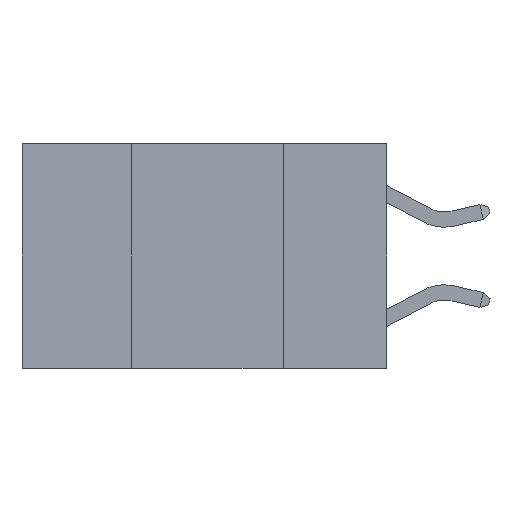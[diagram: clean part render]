
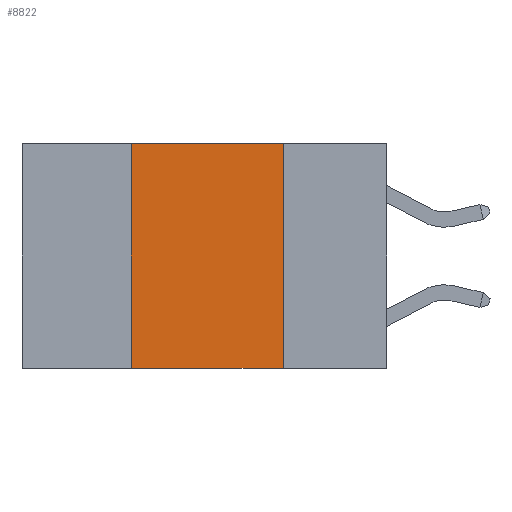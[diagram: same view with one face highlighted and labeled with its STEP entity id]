
A CAD part, left-side view. The second image highlights one B-rep face of the part: STEP entity #8822.
In plain terms, the highlighted planar face has unit normal (-1, 0, 0).
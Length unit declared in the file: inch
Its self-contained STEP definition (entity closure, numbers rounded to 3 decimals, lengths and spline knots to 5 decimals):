
#133 = DIRECTION ( 'NONE',  ( 0., 0., -1. ) ) ;
#435 = VERTEX_POINT ( 'NONE', #14840 ) ;
#555 = VERTEX_POINT ( 'NONE', #12352 ) ;
#850 = LINE ( 'NONE', #15475, #10345 ) ;
#1184 = LINE ( 'NONE', #7112, #5580 ) ;
#1230 = EDGE_LOOP ( 'NONE', ( #7757, #8878, #14988, #6971 ) ) ;
#1262 = EDGE_CURVE ( 'NONE', #16932, #555, #10001, .T. ) ;
#2718 = EDGE_CURVE ( 'NONE', #555, #7319, #850, .T. ) ;
#4563 = VECTOR ( 'NONE', #14627, 39.37008 ) ;
#5580 = VECTOR ( 'NONE', #6818, 39.37008 ) ;
#5904 = VECTOR ( 'NONE', #10977, 39.37008 ) ;
#6214 = CARTESIAN_POINT ( 'NONE',  ( 0., 0.6, -0.37 ) ) ;
#6791 = CARTESIAN_POINT ( 'NONE',  ( 0., 0.6, 0. ) ) ;
#6818 = DIRECTION ( 'NONE',  ( 0., 0., 1. ) ) ;
#6971 = ORIENTED_EDGE ( 'NONE', *, *, #10796, .T. ) ;
#7112 = CARTESIAN_POINT ( 'NONE',  ( 0., 0.42, 0. ) ) ;
#7319 = VERTEX_POINT ( 'NONE', #9051 ) ;
#7757 = ORIENTED_EDGE ( 'NONE', *, *, #2718, .F. ) ;
#8822 = ADVANCED_FACE ( 'NONE', ( #9054 ), #11792, .F. ) ;
#8878 = ORIENTED_EDGE ( 'NONE', *, *, #1262, .F. ) ;
#9051 = CARTESIAN_POINT ( 'NONE',  ( 0., 0.17, -0.37 ) ) ;
#9054 = FACE_OUTER_BOUND ( 'NONE', #1230, .T. ) ;
#10001 = LINE ( 'NONE', #6791, #4563 ) ;
#10232 = DIRECTION ( 'NONE',  ( 1., 0., 0. ) ) ;
#10345 = VECTOR ( 'NONE', #11043, 39.37008 ) ;
#10796 = EDGE_CURVE ( 'NONE', #435, #7319, #15116, .T. ) ;
#10977 = DIRECTION ( 'NONE',  ( 0., -1., 0. ) ) ;
#11043 = DIRECTION ( 'NONE',  ( 0., 0., -1. ) ) ;
#11435 = AXIS2_PLACEMENT_3D ( 'NONE', #17954, #10232, #133 ) ;
#11792 = PLANE ( 'NONE',  #11435 ) ;
#12313 = EDGE_CURVE ( 'NONE', #435, #16932, #1184, .T. ) ;
#12352 = CARTESIAN_POINT ( 'NONE',  ( 0., 0.17, 0. ) ) ;
#14627 = DIRECTION ( 'NONE',  ( 0., -1., 0. ) ) ;
#14760 = CARTESIAN_POINT ( 'NONE',  ( 0., 0.42, 0. ) ) ;
#14840 = CARTESIAN_POINT ( 'NONE',  ( 0., 0.42, -0.37 ) ) ;
#14988 = ORIENTED_EDGE ( 'NONE', *, *, #12313, .F. ) ;
#15116 = LINE ( 'NONE', #6214, #5904 ) ;
#15475 = CARTESIAN_POINT ( 'NONE',  ( 0., 0.17, 0. ) ) ;
#16932 = VERTEX_POINT ( 'NONE', #14760 ) ;
#17954 = CARTESIAN_POINT ( 'NONE',  ( 0., 0.6, 0. ) ) ;
